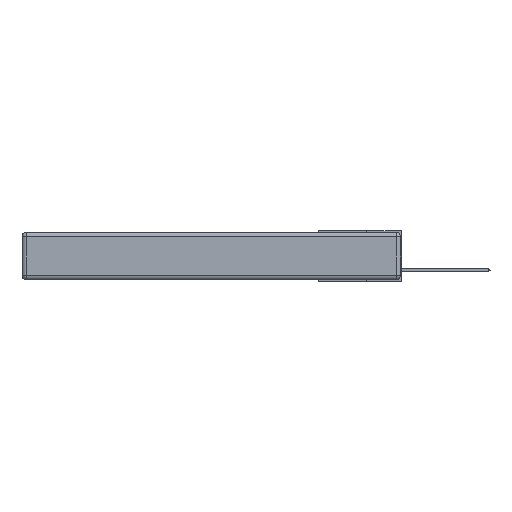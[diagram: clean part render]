
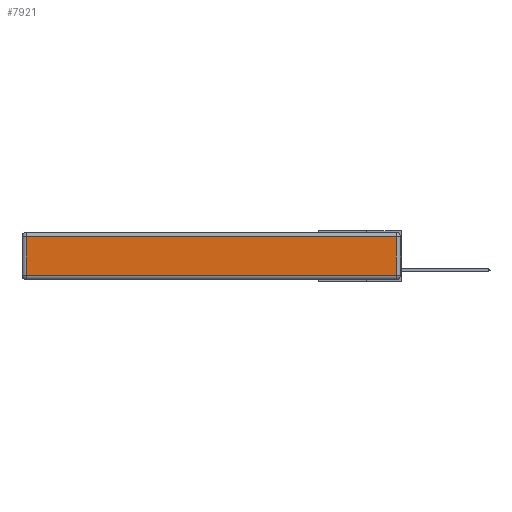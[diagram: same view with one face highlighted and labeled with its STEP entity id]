
A CAD part, left-side view. The second image highlights one B-rep face of the part: STEP entity #7921.
In plain terms, the highlighted planar face has unit normal (-1, 0, 0).
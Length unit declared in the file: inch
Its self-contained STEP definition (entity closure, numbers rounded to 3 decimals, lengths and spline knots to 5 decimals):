
#360 = CARTESIAN_POINT ( 'NONE',  ( 0., 0.03, -0.313 ) ) ;
#816 = EDGE_CURVE ( 'NONE', #1156, #18573, #2411, .T. ) ;
#1036 = EDGE_CURVE ( 'NONE', #18573, #13918, #10676, .T. ) ;
#1156 = VERTEX_POINT ( 'NONE', #5237 ) ;
#2411 = LINE ( 'NONE', #19738, #6413 ) ;
#2739 = EDGE_CURVE ( 'NONE', #15870, #1156, #6435, .T. ) ;
#3815 = DIRECTION ( 'NONE',  ( -1., 0., 0. ) ) ;
#5149 = DIRECTION ( 'NONE',  ( 0., 0., -1. ) ) ;
#5237 = CARTESIAN_POINT ( 'NONE',  ( 0., 0.03, -0.03 ) ) ;
#6084 = EDGE_LOOP ( 'NONE', ( #6869, #23712, #14009, #9862 ) ) ;
#6413 = VECTOR ( 'NONE', #8028, 39.37008 ) ;
#6435 = LINE ( 'NONE', #16963, #21472 ) ;
#6869 = ORIENTED_EDGE ( 'NONE', *, *, #7095, .T. ) ;
#7095 = EDGE_CURVE ( 'NONE', #13918, #15870, #13496, .T. ) ;
#7921 = ADVANCED_FACE ( 'NONE', ( #14394 ), #13412, .T. ) ;
#8028 = DIRECTION ( 'NONE',  ( 0., 1., 0. ) ) ;
#9797 = CARTESIAN_POINT ( 'NONE',  ( 0., 0., -0.313 ) ) ;
#9862 = ORIENTED_EDGE ( 'NONE', *, *, #1036, .T. ) ;
#10676 = LINE ( 'NONE', #24427, #25403 ) ;
#11425 = AXIS2_PLACEMENT_3D ( 'NONE', #19347, #3815, #23449 ) ;
#11839 = DIRECTION ( 'NONE',  ( 0., -1., 0. ) ) ;
#13037 = CARTESIAN_POINT ( 'NONE',  ( 0., 2.72, -0.313 ) ) ;
#13412 = PLANE ( 'NONE',  #11425 ) ;
#13496 = LINE ( 'NONE', #9797, #25160 ) ;
#13918 = VERTEX_POINT ( 'NONE', #13037 ) ;
#14009 = ORIENTED_EDGE ( 'NONE', *, *, #816, .T. ) ;
#14394 = FACE_OUTER_BOUND ( 'NONE', #6084, .T. ) ;
#15870 = VERTEX_POINT ( 'NONE', #360 ) ;
#16963 = CARTESIAN_POINT ( 'NONE',  ( 0., 0.03, -0.343 ) ) ;
#18573 = VERTEX_POINT ( 'NONE', #23448 ) ;
#19347 = CARTESIAN_POINT ( 'NONE',  ( 0., 0., -0.343 ) ) ;
#19738 = CARTESIAN_POINT ( 'NONE',  ( 0., 2.75, -0.03 ) ) ;
#20943 = DIRECTION ( 'NONE',  ( 0., 0., 1. ) ) ;
#21472 = VECTOR ( 'NONE', #20943, 39.37008 ) ;
#23448 = CARTESIAN_POINT ( 'NONE',  ( 0., 2.72, -0.03 ) ) ;
#23449 = DIRECTION ( 'NONE',  ( 0., 0., 1. ) ) ;
#23712 = ORIENTED_EDGE ( 'NONE', *, *, #2739, .T. ) ;
#24427 = CARTESIAN_POINT ( 'NONE',  ( 0., 2.72, -0.343 ) ) ;
#25160 = VECTOR ( 'NONE', #11839, 39.37008 ) ;
#25403 = VECTOR ( 'NONE', #5149, 39.37008 ) ;
